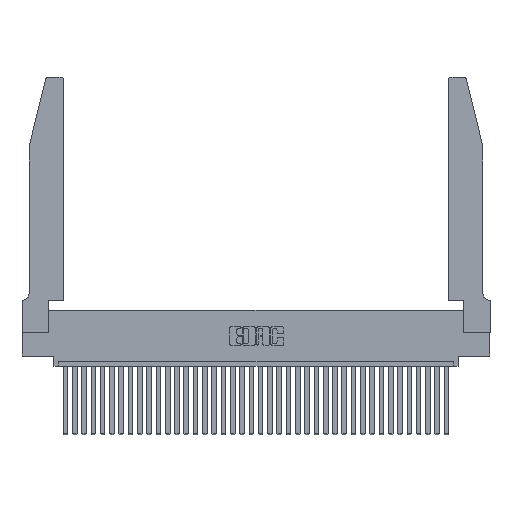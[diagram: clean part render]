
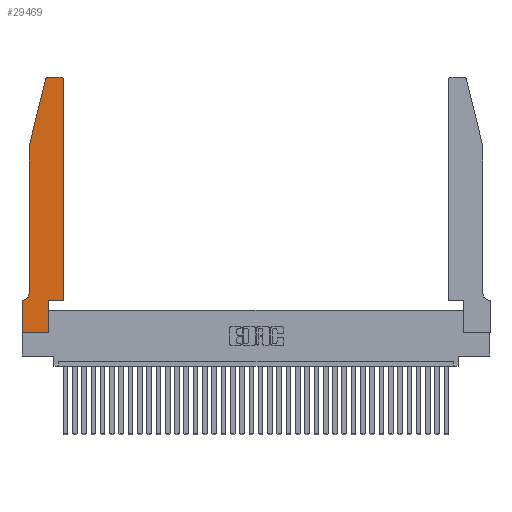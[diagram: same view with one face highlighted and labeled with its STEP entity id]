
A CAD part, top view. The second image highlights one B-rep face of the part: STEP entity #29469.
In plain terms, the highlighted planar face has unit normal (0, 0, 1).
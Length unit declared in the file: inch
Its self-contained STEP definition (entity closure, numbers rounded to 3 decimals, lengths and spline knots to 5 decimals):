
#137 = LINE ( 'NONE', #24724, #12465 ) ;
#197 = CARTESIAN_POINT ( 'NONE',  ( 0.284, 2.72, 0.37 ) ) ;
#204 = VERTEX_POINT ( 'NONE', #31759 ) ;
#949 = CARTESIAN_POINT ( 'NONE',  ( 0.284, 2.75, 0.37 ) ) ;
#1097 = DIRECTION ( 'NONE',  ( 1., 0., 0. ) ) ;
#1369 = LINE ( 'NONE', #6811, #29021 ) ;
#1677 = VERTEX_POINT ( 'NONE', #2374 ) ;
#2374 = CARTESIAN_POINT ( 'NONE',  ( 0.0755, 2., 0.37 ) ) ;
#2387 = ORIENTED_EDGE ( 'NONE', *, *, #35662, .T. ) ;
#2924 = DIRECTION ( 'NONE',  ( 1., 0., 0. ) ) ;
#3118 = VERTEX_POINT ( 'NONE', #19515 ) ;
#3266 = VECTOR ( 'NONE', #34125, 39.37008 ) ;
#3771 = ORIENTED_EDGE ( 'NONE', *, *, #32520, .T. ) ;
#4352 = VERTEX_POINT ( 'NONE', #24722 ) ;
#4624 = EDGE_LOOP ( 'NONE', ( #15729, #31756, #24507, #2387, #5364, #10805, #8336, #27922, #5735, #3771, #36260, #23770 ) ) ;
#4707 = EDGE_CURVE ( 'NONE', #36034, #32123, #6965, .T. ) ;
#5364 = ORIENTED_EDGE ( 'NONE', *, *, #7520, .T. ) ;
#5431 = CARTESIAN_POINT ( 'NONE',  ( 0.0055, 0.42, 0.37 ) ) ;
#5620 = VECTOR ( 'NONE', #20535, 39.37008 ) ;
#5654 = PLANE ( 'NONE',  #7832 ) ;
#5735 = ORIENTED_EDGE ( 'NONE', *, *, #32630, .T. ) ;
#6552 = CARTESIAN_POINT ( 'NONE',  ( 0.0755, 2., 0.37 ) ) ;
#6811 = CARTESIAN_POINT ( 'NONE',  ( 0.2605, 2.75, 0.37 ) ) ;
#6965 = LINE ( 'NONE', #9433, #35911 ) ;
#7108 = AXIS2_PLACEMENT_3D ( 'NONE', #197, #17119, #2924 ) ;
#7520 = EDGE_CURVE ( 'NONE', #4352, #26917, #13394, .T. ) ;
#7832 = AXIS2_PLACEMENT_3D ( 'NONE', #11204, #30482, #33510 ) ;
#7836 = EDGE_CURVE ( 'NONE', #3118, #16388, #13360, .T. ) ;
#8261 = CARTESIAN_POINT ( 'NONE',  ( 0.0755, 2., 0.37 ) ) ;
#8336 = ORIENTED_EDGE ( 'NONE', *, *, #29171, .T. ) ;
#8737 = AXIS2_PLACEMENT_3D ( 'NONE', #5431, #27772, #28015 ) ;
#9433 = CARTESIAN_POINT ( 'NONE',  ( 0., 0., 0.37 ) ) ;
#9675 = VECTOR ( 'NONE', #11919, 39.37008 ) ;
#10116 = LINE ( 'NONE', #34231, #9675 ) ;
#10805 = ORIENTED_EDGE ( 'NONE', *, *, #35331, .T. ) ;
#11204 = CARTESIAN_POINT ( 'NONE',  ( 0., 0.35, 0.37 ) ) ;
#11919 = DIRECTION ( 'NONE',  ( 0., 1., 0. ) ) ;
#12341 = DIRECTION ( 'NONE',  ( 0., 0., 1. ) ) ;
#12465 = VECTOR ( 'NONE', #22110, 39.37008 ) ;
#13245 = VERTEX_POINT ( 'NONE', #949 ) ;
#13360 = CIRCLE ( 'NONE', #31813, 0.03 ) ;
#13394 = CIRCLE ( 'NONE', #8737, 0.07 ) ;
#13826 = VECTOR ( 'NONE', #31487, 39.37008 ) ;
#14481 = CARTESIAN_POINT ( 'NONE',  ( 0., 0., 0.37 ) ) ;
#14596 = VECTOR ( 'NONE', #18925, 39.37008 ) ;
#14686 = LINE ( 'NONE', #6552, #13826 ) ;
#14690 = EDGE_CURVE ( 'NONE', #16388, #13245, #1369, .T. ) ;
#14828 = LINE ( 'NONE', #17575, #5620 ) ;
#14983 = EDGE_CURVE ( 'NONE', #30571, #3118, #10116, .T. ) ;
#15160 = DIRECTION ( 'NONE',  ( -1., 0., 0. ) ) ;
#15276 = DIRECTION ( 'NONE',  ( 1., 0., 0. ) ) ;
#15729 = ORIENTED_EDGE ( 'NONE', *, *, #14690, .T. ) ;
#16388 = VERTEX_POINT ( 'NONE', #33581 ) ;
#17119 = DIRECTION ( 'NONE',  ( 0., 0., 1. ) ) ;
#17575 = CARTESIAN_POINT ( 'NONE',  ( 0.0755, 0.35, 0.37 ) ) ;
#17773 = EDGE_CURVE ( 'NONE', #13245, #28627, #26480, .T. ) ;
#18314 = CARTESIAN_POINT ( 'NONE',  ( 0.25487, 2.72718, 0.37 ) ) ;
#18925 = DIRECTION ( 'NONE',  ( 1., 0., 0. ) ) ;
#19515 = CARTESIAN_POINT ( 'NONE',  ( 0.4505, 2.72, 0.37 ) ) ;
#19785 = EDGE_CURVE ( 'NONE', #28627, #1677, #14686, .T. ) ;
#20535 = DIRECTION ( 'NONE',  ( -1., 0., 0. ) ) ;
#21166 = CARTESIAN_POINT ( 'NONE',  ( 0.4505, 0.35, 0.37 ) ) ;
#22110 = DIRECTION ( 'NONE',  ( 0., 1., 0. ) ) ;
#22965 = LINE ( 'NONE', #35814, #14596 ) ;
#23770 = ORIENTED_EDGE ( 'NONE', *, *, #7836, .T. ) ;
#24507 = ORIENTED_EDGE ( 'NONE', *, *, #19785, .T. ) ;
#24722 = CARTESIAN_POINT ( 'NONE',  ( 0.0755, 0.42, 0.37 ) ) ;
#24724 = CARTESIAN_POINT ( 'NONE',  ( 0.2865, 0.35, 0.37 ) ) ;
#26088 = CARTESIAN_POINT ( 'NONE',  ( 0.4205, 2.72, 0.37 ) ) ;
#26480 = CIRCLE ( 'NONE', #7108, 0.03 ) ;
#26568 = LINE ( 'NONE', #14481, #3266 ) ;
#26917 = VERTEX_POINT ( 'NONE', #32293 ) ;
#27111 = VECTOR ( 'NONE', #27886, 39.37008 ) ;
#27772 = DIRECTION ( 'NONE',  ( 0., 0., -1. ) ) ;
#27886 = DIRECTION ( 'NONE',  ( 0., -1., 0. ) ) ;
#27922 = ORIENTED_EDGE ( 'NONE', *, *, #4707, .T. ) ;
#28015 = DIRECTION ( 'NONE',  ( -1., 0., 0. ) ) ;
#28627 = VERTEX_POINT ( 'NONE', #18314 ) ;
#29021 = VECTOR ( 'NONE', #15160, 39.37008 ) ;
#29171 = EDGE_CURVE ( 'NONE', #31672, #36034, #26568, .T. ) ;
#29192 = CARTESIAN_POINT ( 'NONE',  ( 0., 0.35, 0.37 ) ) ;
#29469 = ADVANCED_FACE ( 'NONE', ( #35914 ), #5654, .T. ) ;
#30482 = DIRECTION ( 'NONE',  ( 0., 0., 1. ) ) ;
#30571 = VERTEX_POINT ( 'NONE', #21166 ) ;
#31487 = DIRECTION ( 'NONE',  ( -0.239, -0.971, 0. ) ) ;
#31672 = VERTEX_POINT ( 'NONE', #29192 ) ;
#31756 = ORIENTED_EDGE ( 'NONE', *, *, #17773, .T. ) ;
#31759 = CARTESIAN_POINT ( 'NONE',  ( 0.2865, 0.35, 0.37 ) ) ;
#31813 = AXIS2_PLACEMENT_3D ( 'NONE', #26088, #12341, #15276 ) ;
#32123 = VERTEX_POINT ( 'NONE', #36330 ) ;
#32293 = CARTESIAN_POINT ( 'NONE',  ( 0.0055, 0.35, 0.37 ) ) ;
#32411 = CARTESIAN_POINT ( 'NONE',  ( 0., 0., 0.37 ) ) ;
#32520 = EDGE_CURVE ( 'NONE', #204, #30571, #22965, .T. ) ;
#32630 = EDGE_CURVE ( 'NONE', #32123, #204, #137, .T. ) ;
#33510 = DIRECTION ( 'NONE',  ( 1., 0., 0. ) ) ;
#33581 = CARTESIAN_POINT ( 'NONE',  ( 0.4205, 2.75, 0.37 ) ) ;
#34119 = LINE ( 'NONE', #8261, #27111 ) ;
#34125 = DIRECTION ( 'NONE',  ( 0., -1., 0. ) ) ;
#34231 = CARTESIAN_POINT ( 'NONE',  ( 0.4505, 0.35, 0.37 ) ) ;
#35331 = EDGE_CURVE ( 'NONE', #26917, #31672, #14828, .T. ) ;
#35662 = EDGE_CURVE ( 'NONE', #1677, #4352, #34119, .T. ) ;
#35814 = CARTESIAN_POINT ( 'NONE',  ( 0.4505, 0.35, 0.37 ) ) ;
#35911 = VECTOR ( 'NONE', #1097, 39.37008 ) ;
#35914 = FACE_OUTER_BOUND ( 'NONE', #4624, .T. ) ;
#36034 = VERTEX_POINT ( 'NONE', #32411 ) ;
#36260 = ORIENTED_EDGE ( 'NONE', *, *, #14983, .T. ) ;
#36330 = CARTESIAN_POINT ( 'NONE',  ( 0.2865, 0., 0.37 ) ) ;
